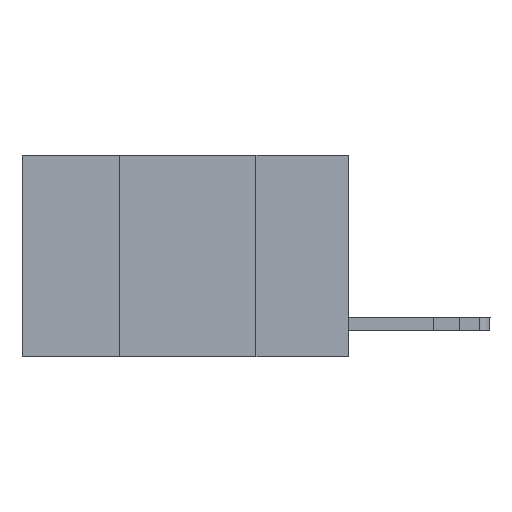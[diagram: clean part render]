
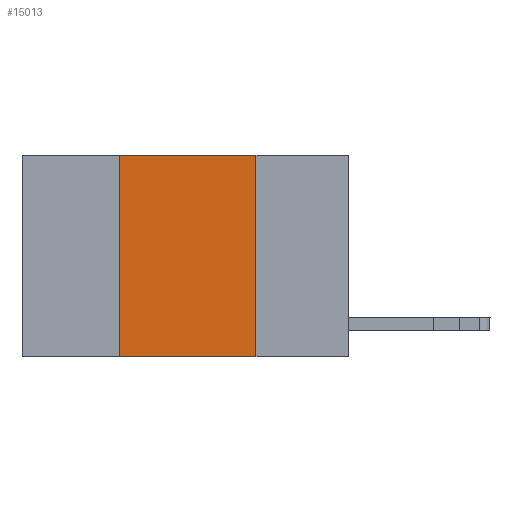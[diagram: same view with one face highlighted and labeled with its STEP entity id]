
A CAD part, left-side view. The second image highlights one B-rep face of the part: STEP entity #15013.
In plain terms, the highlighted planar face has unit normal (-1, 0, 0).
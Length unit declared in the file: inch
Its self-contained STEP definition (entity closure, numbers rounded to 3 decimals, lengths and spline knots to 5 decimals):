
#956 = EDGE_LOOP ( 'NONE', ( #24262, #4163, #6457, #23536 ) ) ;
#983 = EDGE_CURVE ( 'NONE', #3113, #16959, #5634, .T. ) ;
#2055 = DIRECTION ( 'NONE',  ( 0., 0., -1. ) ) ;
#3113 = VERTEX_POINT ( 'NONE', #14186 ) ;
#3408 = FACE_OUTER_BOUND ( 'NONE', #956, .T. ) ;
#3981 = EDGE_CURVE ( 'NONE', #25020, #14110, #13266, .T. ) ;
#4163 = ORIENTED_EDGE ( 'NONE', *, *, #983, .F. ) ;
#5634 = LINE ( 'NONE', #22947, #15611 ) ;
#6457 = ORIENTED_EDGE ( 'NONE', *, *, #17322, .F. ) ;
#6835 = DIRECTION ( 'NONE',  ( 1., 0., 0. ) ) ;
#7874 = LINE ( 'NONE', #16871, #17178 ) ;
#7984 = VECTOR ( 'NONE', #24876, 39.37008 ) ;
#8954 = LINE ( 'NONE', #15909, #24470 ) ;
#10738 = CARTESIAN_POINT ( 'NONE',  ( 0., 0.6, 0. ) ) ;
#13266 = LINE ( 'NONE', #22986, #7984 ) ;
#14110 = VERTEX_POINT ( 'NONE', #23270 ) ;
#14186 = CARTESIAN_POINT ( 'NONE',  ( 0., 0.42, 0. ) ) ;
#14757 = PLANE ( 'NONE',  #19483 ) ;
#15013 = ADVANCED_FACE ( 'NONE', ( #3408 ), #14757, .F. ) ;
#15611 = VECTOR ( 'NONE', #24838, 39.37008 ) ;
#15909 = CARTESIAN_POINT ( 'NONE',  ( 0., 0.17, 0. ) ) ;
#16871 = CARTESIAN_POINT ( 'NONE',  ( 0., 0.42, 0. ) ) ;
#16959 = VERTEX_POINT ( 'NONE', #24941 ) ;
#17178 = VECTOR ( 'NONE', #18761, 39.37008 ) ;
#17322 = EDGE_CURVE ( 'NONE', #25020, #3113, #7874, .T. ) ;
#18761 = DIRECTION ( 'NONE',  ( 0., 0., 1. ) ) ;
#19483 = AXIS2_PLACEMENT_3D ( 'NONE', #10738, #6835, #20566 ) ;
#20566 = DIRECTION ( 'NONE',  ( 0., 0., -1. ) ) ;
#22947 = CARTESIAN_POINT ( 'NONE',  ( 0., 0.6, 0. ) ) ;
#22986 = CARTESIAN_POINT ( 'NONE',  ( 0., 0.6, -0.37 ) ) ;
#23270 = CARTESIAN_POINT ( 'NONE',  ( 0., 0.17, -0.37 ) ) ;
#23536 = ORIENTED_EDGE ( 'NONE', *, *, #3981, .T. ) ;
#24262 = ORIENTED_EDGE ( 'NONE', *, *, #25290, .F. ) ;
#24470 = VECTOR ( 'NONE', #2055, 39.37008 ) ;
#24682 = CARTESIAN_POINT ( 'NONE',  ( 0., 0.42, -0.37 ) ) ;
#24838 = DIRECTION ( 'NONE',  ( 0., -1., 0. ) ) ;
#24876 = DIRECTION ( 'NONE',  ( 0., -1., 0. ) ) ;
#24941 = CARTESIAN_POINT ( 'NONE',  ( 0., 0.17, 0. ) ) ;
#25020 = VERTEX_POINT ( 'NONE', #24682 ) ;
#25290 = EDGE_CURVE ( 'NONE', #16959, #14110, #8954, .T. ) ;
